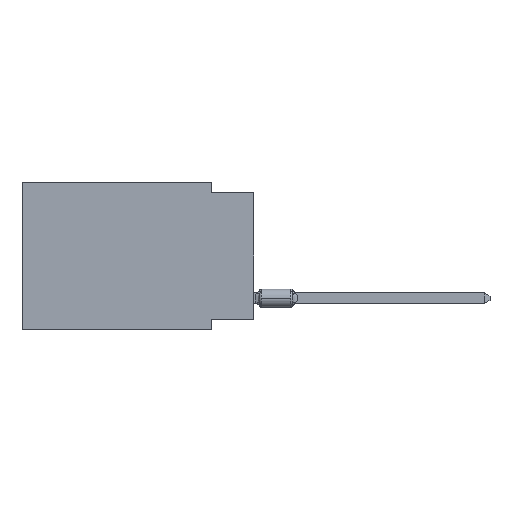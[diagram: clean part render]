
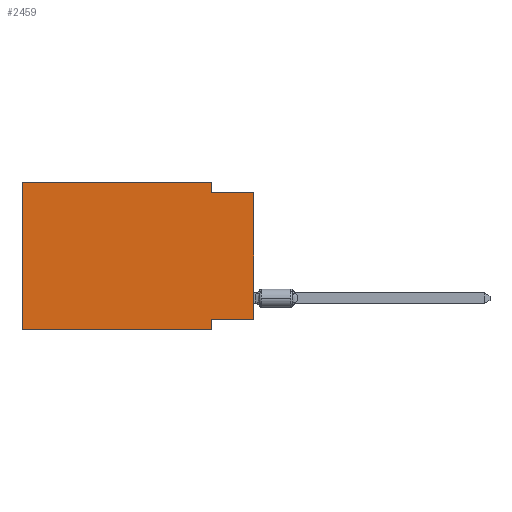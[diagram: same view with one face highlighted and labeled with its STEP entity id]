
A CAD part, left-side view. The second image highlights one B-rep face of the part: STEP entity #2459.
In plain terms, the highlighted planar face has unit normal (-1, 0, 0).
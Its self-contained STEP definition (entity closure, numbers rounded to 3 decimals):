
#70 = ORIENTED_EDGE ( 'NONE', *, *, #6120, .F. ) ;
#112 = DIRECTION ( 'NONE',  ( 1., 0., 0. ) ) ;
#410 = LINE ( 'NONE', #5097, #13102 ) ;
#1289 = ORIENTED_EDGE ( 'NONE', *, *, #11310, .F. ) ;
#1738 = AXIS2_PLACEMENT_3D ( 'NONE', #13538, #112, #4875 ) ;
#1991 = LINE ( 'NONE', #11094, #2999 ) ;
#2289 = CARTESIAN_POINT ( 'NONE',  ( 0., 2.54, -8.255 ) ) ;
#2297 = DIRECTION ( 'NONE',  ( 0., 0., 1. ) ) ;
#2317 = VERTEX_POINT ( 'NONE', #8716 ) ;
#2383 = LINE ( 'NONE', #6504, #12626 ) ;
#2459 = ADVANCED_FACE ( 'NONE', ( #13898 ), #16921, .F. ) ;
#2999 = VECTOR ( 'NONE', #6395, 1000. ) ;
#3389 = VECTOR ( 'NONE', #4574, 1000. ) ;
#4139 = VERTEX_POINT ( 'NONE', #18359 ) ;
#4191 = VERTEX_POINT ( 'NONE', #12123 ) ;
#4315 = EDGE_CURVE ( 'NONE', #15253, #19024, #2383, .T. ) ;
#4488 = LINE ( 'NONE', #10454, #3389 ) ;
#4574 = DIRECTION ( 'NONE',  ( 0., 0., 1. ) ) ;
#4875 = DIRECTION ( 'NONE',  ( 0., 0., -1. ) ) ;
#5097 = CARTESIAN_POINT ( 'NONE',  ( 0., 0., -0.635 ) ) ;
#5187 = LINE ( 'NONE', #7753, #15589 ) ;
#6096 = EDGE_CURVE ( 'NONE', #2317, #4139, #410, .T. ) ;
#6120 = EDGE_CURVE ( 'NONE', #19024, #4191, #5187, .T. ) ;
#6395 = DIRECTION ( 'NONE',  ( 0., -1., 0. ) ) ;
#6504 = CARTESIAN_POINT ( 'NONE',  ( 0., 0., -8.255 ) ) ;
#6662 = DIRECTION ( 'NONE',  ( 0., -1., 0. ) ) ;
#7445 = CARTESIAN_POINT ( 'NONE',  ( 0., 0., -8.255 ) ) ;
#7656 = ORIENTED_EDGE ( 'NONE', *, *, #10218, .F. ) ;
#7753 = CARTESIAN_POINT ( 'NONE',  ( 0., 2.54, -8.89 ) ) ;
#8716 = CARTESIAN_POINT ( 'NONE',  ( 0., 2.54, -0.635 ) ) ;
#9523 = CARTESIAN_POINT ( 'NONE',  ( 0., 13.97, 0. ) ) ;
#9648 = EDGE_LOOP ( 'NONE', ( #17768, #15242, #17239, #7656, #1289, #14522, #70, #17517 ) ) ;
#9843 = CARTESIAN_POINT ( 'NONE',  ( 0., 13.97, 0. ) ) ;
#10139 = LINE ( 'NONE', #9843, #15200 ) ;
#10176 = VECTOR ( 'NONE', #15423, 1000. ) ;
#10218 = EDGE_CURVE ( 'NONE', #19344, #15664, #12375, .T. ) ;
#10454 = CARTESIAN_POINT ( 'NONE',  ( 0., 0., 0. ) ) ;
#10810 = CARTESIAN_POINT ( 'NONE',  ( 0., 2.54, 0. ) ) ;
#11014 = DIRECTION ( 'NONE',  ( 0., 1., 0. ) ) ;
#11094 = CARTESIAN_POINT ( 'NONE',  ( 0., 13.97, -8.89 ) ) ;
#11310 = EDGE_CURVE ( 'NONE', #13148, #19344, #10139, .T. ) ;
#11543 = EDGE_CURVE ( 'NONE', #13148, #4191, #1991, .T. ) ;
#11576 = EDGE_CURVE ( 'NONE', #15664, #2317, #18256, .T. ) ;
#12123 = CARTESIAN_POINT ( 'NONE',  ( 0., 2.54, -8.89 ) ) ;
#12375 = LINE ( 'NONE', #9523, #13490 ) ;
#12626 = VECTOR ( 'NONE', #11014, 1000. ) ;
#13102 = VECTOR ( 'NONE', #6662, 1000. ) ;
#13148 = VERTEX_POINT ( 'NONE', #19017 ) ;
#13385 = CARTESIAN_POINT ( 'NONE',  ( 0., 13.97, 0. ) ) ;
#13490 = VECTOR ( 'NONE', #16782, 1000. ) ;
#13506 = CARTESIAN_POINT ( 'NONE',  ( 0., 2.54, 0. ) ) ;
#13538 = CARTESIAN_POINT ( 'NONE',  ( 0., 13.97, 0. ) ) ;
#13898 = FACE_OUTER_BOUND ( 'NONE', #9648, .T. ) ;
#14522 = ORIENTED_EDGE ( 'NONE', *, *, #11543, .T. ) ;
#15200 = VECTOR ( 'NONE', #2297, 1000. ) ;
#15242 = ORIENTED_EDGE ( 'NONE', *, *, #6096, .F. ) ;
#15253 = VERTEX_POINT ( 'NONE', #7445 ) ;
#15423 = DIRECTION ( 'NONE',  ( 0., 0., -1. ) ) ;
#15589 = VECTOR ( 'NONE', #17038, 1000. ) ;
#15664 = VERTEX_POINT ( 'NONE', #13506 ) ;
#15755 = EDGE_CURVE ( 'NONE', #15253, #4139, #4488, .T. ) ;
#16782 = DIRECTION ( 'NONE',  ( 0., -1., 0. ) ) ;
#16921 = PLANE ( 'NONE',  #1738 ) ;
#17038 = DIRECTION ( 'NONE',  ( 0., 0., -1. ) ) ;
#17239 = ORIENTED_EDGE ( 'NONE', *, *, #11576, .F. ) ;
#17517 = ORIENTED_EDGE ( 'NONE', *, *, #4315, .F. ) ;
#17768 = ORIENTED_EDGE ( 'NONE', *, *, #15755, .T. ) ;
#18256 = LINE ( 'NONE', #10810, #10176 ) ;
#18359 = CARTESIAN_POINT ( 'NONE',  ( 0., 0., -0.635 ) ) ;
#19017 = CARTESIAN_POINT ( 'NONE',  ( 0., 13.97, -8.89 ) ) ;
#19024 = VERTEX_POINT ( 'NONE', #2289 ) ;
#19344 = VERTEX_POINT ( 'NONE', #13385 ) ;
